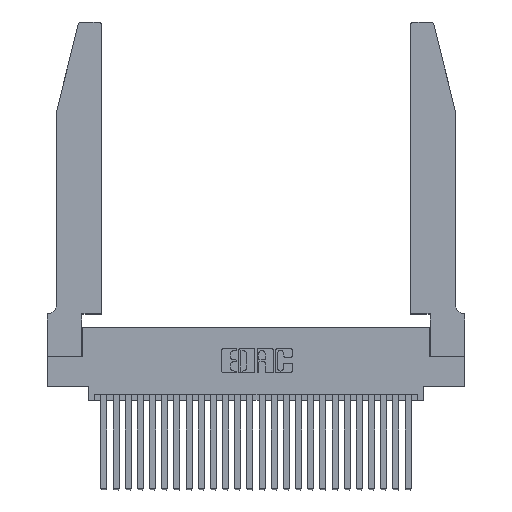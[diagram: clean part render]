
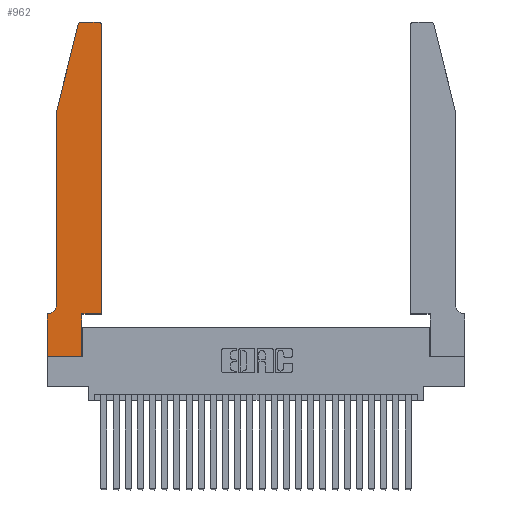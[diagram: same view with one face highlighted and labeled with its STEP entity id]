
A CAD part, top view. The second image highlights one B-rep face of the part: STEP entity #962.
In plain terms, the highlighted planar face has unit normal (0, 0, 1).
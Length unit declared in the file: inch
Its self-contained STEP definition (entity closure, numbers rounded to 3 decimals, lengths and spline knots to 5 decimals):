
#507 = CARTESIAN_POINT ( 'NONE',  ( 0.4205, 2.72, 0.37 ) ) ;
#762 = ORIENTED_EDGE ( 'NONE', *, *, #12110, .T. ) ;
#962 = ADVANCED_FACE ( 'NONE', ( #5548 ), #22249, .T. ) ;
#1089 = ORIENTED_EDGE ( 'NONE', *, *, #11610, .T. ) ;
#1160 = CARTESIAN_POINT ( 'NONE',  ( 0.2605, 2.75, 0.37 ) ) ;
#1568 = DIRECTION ( 'NONE',  ( 0., 1., 0. ) ) ;
#1764 = CARTESIAN_POINT ( 'NONE',  ( 0.284, 2.72, 0.37 ) ) ;
#2064 = DIRECTION ( 'NONE',  ( -0.239, -0.971, 0. ) ) ;
#2238 = LINE ( 'NONE', #8335, #23903 ) ;
#2257 = VERTEX_POINT ( 'NONE', #8973 ) ;
#2444 = EDGE_LOOP ( 'NONE', ( #25088, #10533, #21569, #5572, #22842, #1089, #19290, #8909, #21249, #10872, #762, #12149 ) ) ;
#2740 = DIRECTION ( 'NONE',  ( 1., 0., 0. ) ) ;
#2890 = CARTESIAN_POINT ( 'NONE',  ( 0.2865, 0.35, 0.37 ) ) ;
#3309 = DIRECTION ( 'NONE',  ( 1., 0., 0. ) ) ;
#3408 = VERTEX_POINT ( 'NONE', #4182 ) ;
#3414 = DIRECTION ( 'NONE',  ( -1., 0., 0. ) ) ;
#4042 = DIRECTION ( 'NONE',  ( 1., 0., 0. ) ) ;
#4143 = DIRECTION ( 'NONE',  ( 0., -1., 0. ) ) ;
#4182 = CARTESIAN_POINT ( 'NONE',  ( 0.284, 2.75, 0.37 ) ) ;
#4586 = VECTOR ( 'NONE', #11287, 39.37008 ) ;
#4778 = EDGE_CURVE ( 'NONE', #20538, #14770, #2238, .T. ) ;
#4788 = EDGE_CURVE ( 'NONE', #10274, #10562, #18406, .T. ) ;
#4854 = EDGE_CURVE ( 'NONE', #14595, #10708, #12907, .T. ) ;
#5124 = AXIS2_PLACEMENT_3D ( 'NONE', #507, #15402, #2740 ) ;
#5548 = FACE_OUTER_BOUND ( 'NONE', #2444, .T. ) ;
#5572 = ORIENTED_EDGE ( 'NONE', *, *, #9544, .T. ) ;
#5595 = LINE ( 'NONE', #20577, #22869 ) ;
#5679 = VECTOR ( 'NONE', #3414, 39.37008 ) ;
#5826 = AXIS2_PLACEMENT_3D ( 'NONE', #13815, #20842, #26814 ) ;
#6373 = EDGE_CURVE ( 'NONE', #20656, #9125, #16371, .T. ) ;
#6565 = LINE ( 'NONE', #7622, #12135 ) ;
#7577 = CARTESIAN_POINT ( 'NONE',  ( 0.0055, 0.35, 0.37 ) ) ;
#7622 = CARTESIAN_POINT ( 'NONE',  ( 0.0755, 2., 0.37 ) ) ;
#8320 = CARTESIAN_POINT ( 'NONE',  ( 0.4205, 2.75, 0.37 ) ) ;
#8335 = CARTESIAN_POINT ( 'NONE',  ( 0., 0., 0.37 ) ) ;
#8585 = CARTESIAN_POINT ( 'NONE',  ( 0.2865, 0.35, 0.37 ) ) ;
#8909 = ORIENTED_EDGE ( 'NONE', *, *, #24608, .T. ) ;
#8973 = CARTESIAN_POINT ( 'NONE',  ( 0.4505, 2.72, 0.37 ) ) ;
#9020 = DIRECTION ( 'NONE',  ( -1., 0., 0. ) ) ;
#9125 = VERTEX_POINT ( 'NONE', #8585 ) ;
#9544 = EDGE_CURVE ( 'NONE', #10708, #10274, #6565, .T. ) ;
#9730 = LINE ( 'NONE', #25283, #20098 ) ;
#10236 = DIRECTION ( 'NONE',  ( 1., 0., 0. ) ) ;
#10274 = VERTEX_POINT ( 'NONE', #10816 ) ;
#10533 = ORIENTED_EDGE ( 'NONE', *, *, #10779, .T. ) ;
#10562 = VERTEX_POINT ( 'NONE', #7577 ) ;
#10708 = VERTEX_POINT ( 'NONE', #12227 ) ;
#10710 = CARTESIAN_POINT ( 'NONE',  ( 0.0755, 2., 0.37 ) ) ;
#10779 = EDGE_CURVE ( 'NONE', #3408, #14595, #14668, .T. ) ;
#10798 = VERTEX_POINT ( 'NONE', #8320 ) ;
#10816 = CARTESIAN_POINT ( 'NONE',  ( 0.0755, 0.42, 0.37 ) ) ;
#10872 = ORIENTED_EDGE ( 'NONE', *, *, #18188, .T. ) ;
#10914 = LINE ( 'NONE', #15894, #11547 ) ;
#11287 = DIRECTION ( 'NONE',  ( 0., 1., 0. ) ) ;
#11547 = VECTOR ( 'NONE', #3309, 39.37008 ) ;
#11610 = EDGE_CURVE ( 'NONE', #10562, #20538, #22089, .T. ) ;
#12110 = EDGE_CURVE ( 'NONE', #12931, #2257, #9730, .T. ) ;
#12135 = VECTOR ( 'NONE', #13915, 39.37008 ) ;
#12149 = ORIENTED_EDGE ( 'NONE', *, *, #14468, .T. ) ;
#12227 = CARTESIAN_POINT ( 'NONE',  ( 0.0755, 2., 0.37 ) ) ;
#12607 = CARTESIAN_POINT ( 'NONE',  ( 0.0055, 0.42, 0.37 ) ) ;
#12907 = LINE ( 'NONE', #10710, #22628 ) ;
#12931 = VERTEX_POINT ( 'NONE', #24153 ) ;
#13680 = CARTESIAN_POINT ( 'NONE',  ( 0.25487, 2.72718, 0.37 ) ) ;
#13815 = CARTESIAN_POINT ( 'NONE',  ( 0., 0.35, 0.37 ) ) ;
#13915 = DIRECTION ( 'NONE',  ( 0., -1., 0. ) ) ;
#14468 = EDGE_CURVE ( 'NONE', #2257, #10798, #21790, .T. ) ;
#14595 = VERTEX_POINT ( 'NONE', #13680 ) ;
#14668 = CIRCLE ( 'NONE', #24782, 0.03 ) ;
#14691 = DIRECTION ( 'NONE',  ( -1., 0., 0. ) ) ;
#14770 = VERTEX_POINT ( 'NONE', #20384 ) ;
#15402 = DIRECTION ( 'NONE',  ( 0., 0., 1. ) ) ;
#15703 = CARTESIAN_POINT ( 'NONE',  ( 0.2865, 0., 0.37 ) ) ;
#15894 = CARTESIAN_POINT ( 'NONE',  ( 0., 0., 0.37 ) ) ;
#16371 = LINE ( 'NONE', #2890, #4586 ) ;
#16580 = DIRECTION ( 'NONE',  ( 0., 0., 1. ) ) ;
#16783 = LINE ( 'NONE', #1160, #5679 ) ;
#16805 = EDGE_CURVE ( 'NONE', #10798, #3408, #16783, .T. ) ;
#17275 = CARTESIAN_POINT ( 'NONE',  ( 0.0755, 0.35, 0.37 ) ) ;
#18188 = EDGE_CURVE ( 'NONE', #9125, #12931, #5595, .T. ) ;
#18406 = CIRCLE ( 'NONE', #21955, 0.07 ) ;
#19290 = ORIENTED_EDGE ( 'NONE', *, *, #4778, .T. ) ;
#20098 = VECTOR ( 'NONE', #1568, 39.37008 ) ;
#20384 = CARTESIAN_POINT ( 'NONE',  ( 0., 0., 0.37 ) ) ;
#20538 = VERTEX_POINT ( 'NONE', #21540 ) ;
#20577 = CARTESIAN_POINT ( 'NONE',  ( 0.4505, 0.35, 0.37 ) ) ;
#20656 = VERTEX_POINT ( 'NONE', #15703 ) ;
#20842 = DIRECTION ( 'NONE',  ( 0., 0., 1. ) ) ;
#21249 = ORIENTED_EDGE ( 'NONE', *, *, #6373, .T. ) ;
#21540 = CARTESIAN_POINT ( 'NONE',  ( 0., 0.35, 0.37 ) ) ;
#21569 = ORIENTED_EDGE ( 'NONE', *, *, #4854, .T. ) ;
#21790 = CIRCLE ( 'NONE', #5124, 0.03 ) ;
#21955 = AXIS2_PLACEMENT_3D ( 'NONE', #12607, #27070, #14691 ) ;
#22089 = LINE ( 'NONE', #17275, #26921 ) ;
#22249 = PLANE ( 'NONE',  #5826 ) ;
#22628 = VECTOR ( 'NONE', #2064, 39.37008 ) ;
#22842 = ORIENTED_EDGE ( 'NONE', *, *, #4788, .T. ) ;
#22869 = VECTOR ( 'NONE', #10236, 39.37008 ) ;
#23903 = VECTOR ( 'NONE', #4143, 39.37008 ) ;
#24153 = CARTESIAN_POINT ( 'NONE',  ( 0.4505, 0.35, 0.37 ) ) ;
#24608 = EDGE_CURVE ( 'NONE', #14770, #20656, #10914, .T. ) ;
#24782 = AXIS2_PLACEMENT_3D ( 'NONE', #1764, #16580, #4042 ) ;
#25088 = ORIENTED_EDGE ( 'NONE', *, *, #16805, .T. ) ;
#25283 = CARTESIAN_POINT ( 'NONE',  ( 0.4505, 0.35, 0.37 ) ) ;
#26814 = DIRECTION ( 'NONE',  ( 1., 0., 0. ) ) ;
#26921 = VECTOR ( 'NONE', #9020, 39.37008 ) ;
#27070 = DIRECTION ( 'NONE',  ( 0., 0., -1. ) ) ;
